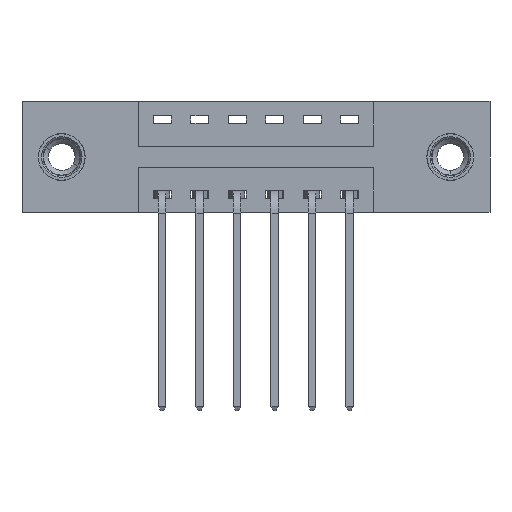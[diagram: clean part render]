
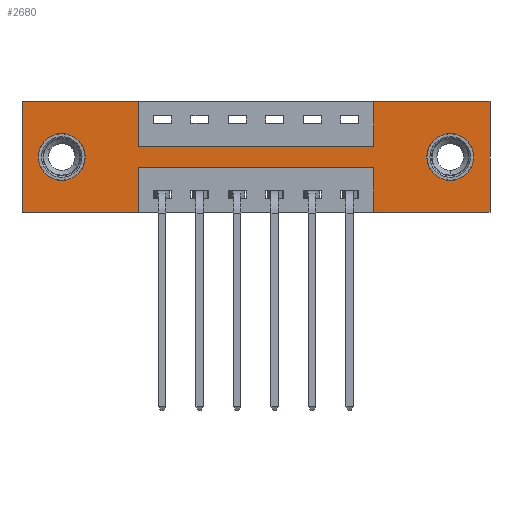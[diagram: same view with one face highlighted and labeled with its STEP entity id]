
A CAD part, front view. The second image highlights one B-rep face of the part: STEP entity #2680.
In plain terms, the highlighted planar face has unit normal (0, -1, 0).
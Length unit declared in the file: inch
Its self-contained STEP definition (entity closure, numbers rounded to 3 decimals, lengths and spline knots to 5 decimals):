
#10 = VERTEX_POINT ( 'NONE', #6213 ) ;
#28 = LINE ( 'NONE', #7863, #1332 ) ;
#211 = LINE ( 'NONE', #5315, #6242 ) ;
#497 = LINE ( 'NONE', #9095, #4715 ) ;
#524 = EDGE_CURVE ( 'NONE', #4476, #1030, #3907, .T. ) ;
#583 = CIRCLE ( 'NONE', #5629, 0.078 ) ;
#635 = CARTESIAN_POINT ( 'NONE',  ( 1.1725, 0., -0.15 ) ) ;
#638 = VERTEX_POINT ( 'NONE', #8386 ) ;
#688 = VERTEX_POINT ( 'NONE', #2191 ) ;
#862 = VECTOR ( 'NONE', #6410, 39.37008 ) ;
#1030 = VERTEX_POINT ( 'NONE', #4569 ) ;
#1035 = AXIS2_PLACEMENT_3D ( 'NONE', #1927, #7259, #2776 ) ;
#1146 = DIRECTION ( 'NONE',  ( 0., 0., -1. ) ) ;
#1149 = VERTEX_POINT ( 'NONE', #2039 ) ;
#1255 = VERTEX_POINT ( 'NONE', #3839 ) ;
#1332 = VECTOR ( 'NONE', #8603, 39.37008 ) ;
#1393 = CARTESIAN_POINT ( 'NONE',  ( 1.1725, 0., -0.22 ) ) ;
#1428 = CARTESIAN_POINT ( 'NONE',  ( 0.1325, 0., -0.263 ) ) ;
#1500 = LINE ( 'NONE', #3860, #5435 ) ;
#1562 = DIRECTION ( 'NONE',  ( 0., 1., 0. ) ) ;
#1684 = DIRECTION ( 'NONE',  ( 0., 1., 0. ) ) ;
#1783 = AXIS2_PLACEMENT_3D ( 'NONE', #6328, #1684, #7045 ) ;
#1812 = VERTEX_POINT ( 'NONE', #6816 ) ;
#1832 = EDGE_LOOP ( 'NONE', ( #6761, #6771 ) ) ;
#1869 = LINE ( 'NONE', #5610, #9618 ) ;
#1927 = CARTESIAN_POINT ( 'NONE',  ( 1.4275, 0., -0.185 ) ) ;
#2039 = CARTESIAN_POINT ( 'NONE',  ( 1.4275, 0., -0.107 ) ) ;
#2103 = DIRECTION ( 'NONE',  ( 0., 1., 0. ) ) ;
#2190 = VERTEX_POINT ( 'NONE', #5772 ) ;
#2191 = CARTESIAN_POINT ( 'NONE',  ( 1.56, 0., -0.37 ) ) ;
#2260 = DIRECTION ( 'NONE',  ( 1., 0., 0. ) ) ;
#2281 = EDGE_LOOP ( 'NONE', ( #6036, #6751 ) ) ;
#2378 = CARTESIAN_POINT ( 'NONE',  ( 1.56, 0., 0. ) ) ;
#2398 = EDGE_CURVE ( 'NONE', #6042, #7601, #583, .T. ) ;
#2589 = CIRCLE ( 'NONE', #1783, 0.078 ) ;
#2680 = ADVANCED_FACE ( 'NONE', ( #3252, #3471, #4080 ), #8448, .T. ) ;
#2776 = DIRECTION ( 'NONE',  ( 0., 0., -1. ) ) ;
#2826 = EDGE_CURVE ( 'NONE', #1030, #6594, #28, .T. ) ;
#2951 = EDGE_CURVE ( 'NONE', #1255, #1149, #9287, .T. ) ;
#3075 = DIRECTION ( 'NONE',  ( -1., 0., 0. ) ) ;
#3100 = DIRECTION ( 'NONE',  ( 0., 0., -1. ) ) ;
#3252 = FACE_BOUND ( 'NONE', #2281, .T. ) ;
#3322 = VECTOR ( 'NONE', #3075, 39.37008 ) ;
#3336 = CARTESIAN_POINT ( 'NONE',  ( 0.3875, 0., -0.22 ) ) ;
#3471 = FACE_BOUND ( 'NONE', #1832, .T. ) ;
#3779 = VECTOR ( 'NONE', #5798, 39.37008 ) ;
#3839 = CARTESIAN_POINT ( 'NONE',  ( 1.4275, 0., -0.263 ) ) ;
#3858 = EDGE_CURVE ( 'NONE', #2190, #4476, #1500, .T. ) ;
#3860 = CARTESIAN_POINT ( 'NONE',  ( 0.3875, 0., -0.15 ) ) ;
#3907 = LINE ( 'NONE', #4396, #3779 ) ;
#3921 = EDGE_CURVE ( 'NONE', #7601, #6042, #6903, .T. ) ;
#3930 = EDGE_CURVE ( 'NONE', #10, #4104, #497, .T. ) ;
#4080 = FACE_OUTER_BOUND ( 'NONE', #5513, .T. ) ;
#4099 = DIRECTION ( 'NONE',  ( 0., 0., 1. ) ) ;
#4104 = VERTEX_POINT ( 'NONE', #8779 ) ;
#4116 = DIRECTION ( 'NONE',  ( -1., 0., 0. ) ) ;
#4134 = CARTESIAN_POINT ( 'NONE',  ( 0., 0., -0.37 ) ) ;
#4144 = VERTEX_POINT ( 'NONE', #7363 ) ;
#4145 = LINE ( 'NONE', #2378, #9738 ) ;
#4396 = CARTESIAN_POINT ( 'NONE',  ( 1.1725, 0., 0. ) ) ;
#4454 = EDGE_CURVE ( 'NONE', #8752, #10, #211, .T. ) ;
#4476 = VERTEX_POINT ( 'NONE', #635 ) ;
#4569 = CARTESIAN_POINT ( 'NONE',  ( 1.1725, 0., 0. ) ) ;
#4715 = VECTOR ( 'NONE', #4748, 39.37008 ) ;
#4748 = DIRECTION ( 'NONE',  ( 1., 0., 0. ) ) ;
#4800 = CARTESIAN_POINT ( 'NONE',  ( 0., 0., -0.37 ) ) ;
#4971 = VERTEX_POINT ( 'NONE', #1393 ) ;
#5028 = EDGE_CURVE ( 'NONE', #4104, #2190, #5428, .T. ) ;
#5190 = AXIS2_PLACEMENT_3D ( 'NONE', #6227, #1562, #6936 ) ;
#5281 = DIRECTION ( 'NONE',  ( 0., -1., 0. ) ) ;
#5284 = EDGE_CURVE ( 'NONE', #688, #638, #7019, .T. ) ;
#5315 = CARTESIAN_POINT ( 'NONE',  ( 0., 0., 0. ) ) ;
#5362 = LINE ( 'NONE', #6109, #3322 ) ;
#5428 = LINE ( 'NONE', #6130, #9033 ) ;
#5435 = VECTOR ( 'NONE', #2260, 39.37008 ) ;
#5447 = LINE ( 'NONE', #3336, #7594 ) ;
#5513 = EDGE_LOOP ( 'NONE', ( #6808, #6848, #6888, #6902, #7145, #7167, #7695, #7804, #7867, #8201, #8219, #8682 ) ) ;
#5572 = DIRECTION ( 'NONE',  ( 0., 0., -1. ) ) ;
#5597 = LINE ( 'NONE', #5833, #9189 ) ;
#5610 = CARTESIAN_POINT ( 'NONE',  ( 1.1725, 0., -0.37 ) ) ;
#5629 = AXIS2_PLACEMENT_3D ( 'NONE', #6712, #2103, #7420 ) ;
#5772 = CARTESIAN_POINT ( 'NONE',  ( 0.3875, 0., -0.15 ) ) ;
#5798 = DIRECTION ( 'NONE',  ( 0., 0., 1. ) ) ;
#5833 = CARTESIAN_POINT ( 'NONE',  ( 0.3875, 0., -0.37 ) ) ;
#5950 = AXIS2_PLACEMENT_3D ( 'NONE', #4800, #5281, #5572 ) ;
#6036 = ORIENTED_EDGE ( 'NONE', *, *, #7261, .T. ) ;
#6042 = VERTEX_POINT ( 'NONE', #9396 ) ;
#6085 = DIRECTION ( 'NONE',  ( 0., 0., 1. ) ) ;
#6109 = CARTESIAN_POINT ( 'NONE',  ( 0., 0., -0.37 ) ) ;
#6130 = CARTESIAN_POINT ( 'NONE',  ( 0.3875, 0., 0. ) ) ;
#6213 = CARTESIAN_POINT ( 'NONE',  ( 0., 0., 0. ) ) ;
#6227 = CARTESIAN_POINT ( 'NONE',  ( 0.1325, 0., -0.185 ) ) ;
#6242 = VECTOR ( 'NONE', #6085, 39.37008 ) ;
#6328 = CARTESIAN_POINT ( 'NONE',  ( 1.4275, 0., -0.185 ) ) ;
#6410 = DIRECTION ( 'NONE',  ( -1., 0., 0. ) ) ;
#6594 = VERTEX_POINT ( 'NONE', #8589 ) ;
#6712 = CARTESIAN_POINT ( 'NONE',  ( 0.1325, 0., -0.185 ) ) ;
#6751 = ORIENTED_EDGE ( 'NONE', *, *, #2951, .T. ) ;
#6761 = ORIENTED_EDGE ( 'NONE', *, *, #2398, .T. ) ;
#6771 = ORIENTED_EDGE ( 'NONE', *, *, #3921, .T. ) ;
#6808 = ORIENTED_EDGE ( 'NONE', *, *, #8003, .F. ) ;
#6816 = CARTESIAN_POINT ( 'NONE',  ( 0.3875, 0., -0.37 ) ) ;
#6848 = ORIENTED_EDGE ( 'NONE', *, *, #9080, .F. ) ;
#6888 = ORIENTED_EDGE ( 'NONE', *, *, #9692, .F. ) ;
#6902 = ORIENTED_EDGE ( 'NONE', *, *, #5284, .F. ) ;
#6903 = CIRCLE ( 'NONE', #5190, 0.078 ) ;
#6936 = DIRECTION ( 'NONE',  ( 0., 0., 1. ) ) ;
#7019 = LINE ( 'NONE', #4134, #862 ) ;
#7045 = DIRECTION ( 'NONE',  ( 0., 0., -1. ) ) ;
#7145 = ORIENTED_EDGE ( 'NONE', *, *, #8984, .F. ) ;
#7167 = ORIENTED_EDGE ( 'NONE', *, *, #2826, .F. ) ;
#7259 = DIRECTION ( 'NONE',  ( 0., 1., 0. ) ) ;
#7261 = EDGE_CURVE ( 'NONE', #1149, #1255, #2589, .T. ) ;
#7363 = CARTESIAN_POINT ( 'NONE',  ( 0.3875, 0., -0.22 ) ) ;
#7420 = DIRECTION ( 'NONE',  ( 0., 0., 1. ) ) ;
#7594 = VECTOR ( 'NONE', #4116, 39.37008 ) ;
#7601 = VERTEX_POINT ( 'NONE', #1428 ) ;
#7607 = EDGE_CURVE ( 'NONE', #1812, #8752, #5362, .T. ) ;
#7665 = DIRECTION ( 'NONE',  ( 0., 0., -1. ) ) ;
#7695 = ORIENTED_EDGE ( 'NONE', *, *, #524, .F. ) ;
#7804 = ORIENTED_EDGE ( 'NONE', *, *, #3858, .F. ) ;
#7863 = CARTESIAN_POINT ( 'NONE',  ( 0., 0., 0. ) ) ;
#7867 = ORIENTED_EDGE ( 'NONE', *, *, #5028, .F. ) ;
#8003 = EDGE_CURVE ( 'NONE', #4144, #1812, #5597, .T. ) ;
#8201 = ORIENTED_EDGE ( 'NONE', *, *, #3930, .F. ) ;
#8219 = ORIENTED_EDGE ( 'NONE', *, *, #4454, .F. ) ;
#8386 = CARTESIAN_POINT ( 'NONE',  ( 1.1725, 0., -0.37 ) ) ;
#8448 = PLANE ( 'NONE',  #5950 ) ;
#8589 = CARTESIAN_POINT ( 'NONE',  ( 1.56, 0., 0. ) ) ;
#8603 = DIRECTION ( 'NONE',  ( 1., 0., 0. ) ) ;
#8682 = ORIENTED_EDGE ( 'NONE', *, *, #7607, .F. ) ;
#8752 = VERTEX_POINT ( 'NONE', #9566 ) ;
#8779 = CARTESIAN_POINT ( 'NONE',  ( 0.3875, 0., 0. ) ) ;
#8984 = EDGE_CURVE ( 'NONE', #6594, #688, #4145, .T. ) ;
#9033 = VECTOR ( 'NONE', #3100, 39.37008 ) ;
#9080 = EDGE_CURVE ( 'NONE', #4971, #4144, #5447, .T. ) ;
#9095 = CARTESIAN_POINT ( 'NONE',  ( 0., 0., 0. ) ) ;
#9189 = VECTOR ( 'NONE', #1146, 39.37008 ) ;
#9287 = CIRCLE ( 'NONE', #1035, 0.078 ) ;
#9396 = CARTESIAN_POINT ( 'NONE',  ( 0.1325, 0., -0.107 ) ) ;
#9566 = CARTESIAN_POINT ( 'NONE',  ( 0., 0., -0.37 ) ) ;
#9618 = VECTOR ( 'NONE', #4099, 39.37008 ) ;
#9692 = EDGE_CURVE ( 'NONE', #638, #4971, #1869, .T. ) ;
#9738 = VECTOR ( 'NONE', #7665, 39.37008 ) ;
